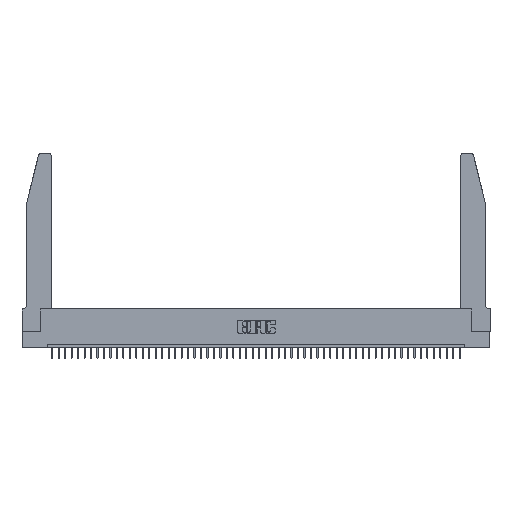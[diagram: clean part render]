
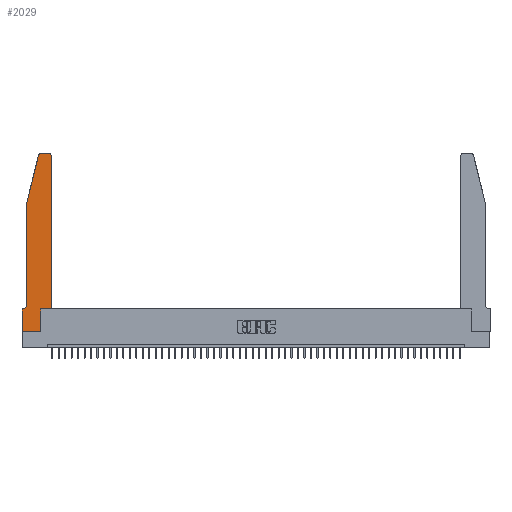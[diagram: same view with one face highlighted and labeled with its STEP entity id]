
A CAD part, top view. The second image highlights one B-rep face of the part: STEP entity #2029.
In plain terms, the highlighted planar face has unit normal (0, 0, 1).
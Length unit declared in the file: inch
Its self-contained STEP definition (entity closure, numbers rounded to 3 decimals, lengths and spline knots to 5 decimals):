
#716 = AXIS2_PLACEMENT_3D ( 'NONE', #21433, #33277, #48469 ) ;
#717 = CARTESIAN_POINT ( 'NONE',  ( 0.4505, 0.35, 0.37 ) ) ;
#1204 = AXIS2_PLACEMENT_3D ( 'NONE', #40837, #10070, #17505 ) ;
#1497 = DIRECTION ( 'NONE',  ( -0.239, -0.971, 0. ) ) ;
#2029 = ADVANCED_FACE ( 'NONE', ( #33065 ), #3967, .T. ) ;
#2465 = EDGE_CURVE ( 'NONE', #15066, #14493, #23351, .T. ) ;
#3002 = VECTOR ( 'NONE', #42410, 39.37008 ) ;
#3051 = ORIENTED_EDGE ( 'NONE', *, *, #10508, .T. ) ;
#3434 = LINE ( 'NONE', #7580, #43894 ) ;
#3967 = PLANE ( 'NONE',  #37011 ) ;
#4148 = DIRECTION ( 'NONE',  ( 1., 0., 0. ) ) ;
#4444 = DIRECTION ( 'NONE',  ( 1., 0., 0. ) ) ;
#4973 = EDGE_CURVE ( 'NONE', #5153, #47117, #19461, .T. ) ;
#5054 = CARTESIAN_POINT ( 'NONE',  ( 0.0755, 2., 0.37 ) ) ;
#5062 = EDGE_CURVE ( 'NONE', #17754, #27883, #32787, .T. ) ;
#5153 = VERTEX_POINT ( 'NONE', #25696 ) ;
#5243 = CARTESIAN_POINT ( 'NONE',  ( 0.4505, 2.72, 0.37 ) ) ;
#5812 = EDGE_CURVE ( 'NONE', #46276, #41531, #23033, .T. ) ;
#6817 = LINE ( 'NONE', #15772, #7453 ) ;
#6867 = CARTESIAN_POINT ( 'NONE',  ( 0., 0.35, 0.37 ) ) ;
#7453 = VECTOR ( 'NONE', #4148, 39.37008 ) ;
#7580 = CARTESIAN_POINT ( 'NONE',  ( 0.2865, 0.35, 0.37 ) ) ;
#7877 = EDGE_LOOP ( 'NONE', ( #15060, #33565, #18424, #22862, #23961, #18065, #3051, #20546, #26786, #35140, #23641, #13980 ) ) ;
#8109 = VECTOR ( 'NONE', #30104, 39.37008 ) ;
#9241 = CARTESIAN_POINT ( 'NONE',  ( 0.2865, 0., 0.37 ) ) ;
#9761 = VECTOR ( 'NONE', #30238, 39.37008 ) ;
#10070 = DIRECTION ( 'NONE',  ( 0., 0., 1. ) ) ;
#10508 = EDGE_CURVE ( 'NONE', #20552, #17754, #45539, .T. ) ;
#11319 = CARTESIAN_POINT ( 'NONE',  ( 0.0755, 0.35, 0.37 ) ) ;
#11421 = DIRECTION ( 'NONE',  ( 0., 1., 0. ) ) ;
#11685 = CARTESIAN_POINT ( 'NONE',  ( 0.4205, 2.75, 0.37 ) ) ;
#12059 = EDGE_CURVE ( 'NONE', #37033, #20552, #33812, .T. ) ;
#12206 = VECTOR ( 'NONE', #31632, 39.37008 ) ;
#12526 = DIRECTION ( 'NONE',  ( 0., 0., 1. ) ) ;
#13980 = ORIENTED_EDGE ( 'NONE', *, *, #49654, .T. ) ;
#14331 = AXIS2_PLACEMENT_3D ( 'NONE', #43253, #12526, #39569 ) ;
#14355 = EDGE_CURVE ( 'NONE', #41531, #37033, #35327, .T. ) ;
#14493 = VERTEX_POINT ( 'NONE', #34597 ) ;
#15060 = ORIENTED_EDGE ( 'NONE', *, *, #40405, .T. ) ;
#15066 = VERTEX_POINT ( 'NONE', #41230 ) ;
#15756 = CARTESIAN_POINT ( 'NONE',  ( 0.2865, 0.35, 0.37 ) ) ;
#15772 = CARTESIAN_POINT ( 'NONE',  ( 0.4505, 0.35, 0.37 ) ) ;
#16416 = VECTOR ( 'NONE', #36017, 39.37008 ) ;
#17505 = DIRECTION ( 'NONE',  ( 1., 0., 0. ) ) ;
#17594 = CARTESIAN_POINT ( 'NONE',  ( 0.0755, 0.42, 0.37 ) ) ;
#17754 = VERTEX_POINT ( 'NONE', #36945 ) ;
#18065 = ORIENTED_EDGE ( 'NONE', *, *, #12059, .T. ) ;
#18085 = CARTESIAN_POINT ( 'NONE',  ( 0., 0., 0.37 ) ) ;
#18424 = ORIENTED_EDGE ( 'NONE', *, *, #18780, .T. ) ;
#18780 = EDGE_CURVE ( 'NONE', #14493, #46276, #29646, .T. ) ;
#19461 = LINE ( 'NONE', #717, #12206 ) ;
#20546 = ORIENTED_EDGE ( 'NONE', *, *, #5062, .T. ) ;
#20552 = VERTEX_POINT ( 'NONE', #21061 ) ;
#21061 = CARTESIAN_POINT ( 'NONE',  ( 0., 0.35, 0.37 ) ) ;
#21070 = EDGE_CURVE ( 'NONE', #27883, #24207, #3434, .T. ) ;
#21433 = CARTESIAN_POINT ( 'NONE',  ( 0.0055, 0.42, 0.37 ) ) ;
#22862 = ORIENTED_EDGE ( 'NONE', *, *, #5812, .T. ) ;
#23033 = LINE ( 'NONE', #41065, #9761 ) ;
#23179 = CARTESIAN_POINT ( 'NONE',  ( 0.2605, 2.75, 0.37 ) ) ;
#23351 = CIRCLE ( 'NONE', #14331, 0.03 ) ;
#23486 = EDGE_CURVE ( 'NONE', #24207, #5153, #6817, .T. ) ;
#23641 = ORIENTED_EDGE ( 'NONE', *, *, #4973, .T. ) ;
#23961 = ORIENTED_EDGE ( 'NONE', *, *, #14355, .T. ) ;
#24207 = VERTEX_POINT ( 'NONE', #15756 ) ;
#25696 = CARTESIAN_POINT ( 'NONE',  ( 0.4505, 0.35, 0.37 ) ) ;
#25929 = VERTEX_POINT ( 'NONE', #11685 ) ;
#26786 = ORIENTED_EDGE ( 'NONE', *, *, #21070, .T. ) ;
#27883 = VERTEX_POINT ( 'NONE', #9241 ) ;
#27953 = CARTESIAN_POINT ( 'NONE',  ( 0.0755, 2., 0.37 ) ) ;
#29646 = LINE ( 'NONE', #5054, #48946 ) ;
#30104 = DIRECTION ( 'NONE',  ( 0., -1., 0. ) ) ;
#30238 = DIRECTION ( 'NONE',  ( 0., -1., 0. ) ) ;
#30823 = VECTOR ( 'NONE', #46492, 39.37008 ) ;
#31632 = DIRECTION ( 'NONE',  ( 0., 1., 0. ) ) ;
#32631 = CIRCLE ( 'NONE', #1204, 0.03 ) ;
#32685 = CARTESIAN_POINT ( 'NONE',  ( 0.0055, 0.35, 0.37 ) ) ;
#32787 = LINE ( 'NONE', #32802, #16416 ) ;
#32802 = CARTESIAN_POINT ( 'NONE',  ( 0., 0., 0.37 ) ) ;
#33065 = FACE_OUTER_BOUND ( 'NONE', #7877, .T. ) ;
#33277 = DIRECTION ( 'NONE',  ( 0., 0., -1. ) ) ;
#33565 = ORIENTED_EDGE ( 'NONE', *, *, #2465, .T. ) ;
#33812 = LINE ( 'NONE', #11319, #3002 ) ;
#34597 = CARTESIAN_POINT ( 'NONE',  ( 0.25487, 2.72718, 0.37 ) ) ;
#35140 = ORIENTED_EDGE ( 'NONE', *, *, #23486, .T. ) ;
#35327 = CIRCLE ( 'NONE', #716, 0.07 ) ;
#36017 = DIRECTION ( 'NONE',  ( 1., 0., 0. ) ) ;
#36945 = CARTESIAN_POINT ( 'NONE',  ( 0., 0., 0.37 ) ) ;
#37011 = AXIS2_PLACEMENT_3D ( 'NONE', #6867, #48192, #4444 ) ;
#37033 = VERTEX_POINT ( 'NONE', #32685 ) ;
#39569 = DIRECTION ( 'NONE',  ( 1., 0., 0. ) ) ;
#40405 = EDGE_CURVE ( 'NONE', #25929, #15066, #41118, .T. ) ;
#40837 = CARTESIAN_POINT ( 'NONE',  ( 0.4205, 2.72, 0.37 ) ) ;
#41065 = CARTESIAN_POINT ( 'NONE',  ( 0.0755, 2., 0.37 ) ) ;
#41118 = LINE ( 'NONE', #23179, #30823 ) ;
#41230 = CARTESIAN_POINT ( 'NONE',  ( 0.284, 2.75, 0.37 ) ) ;
#41531 = VERTEX_POINT ( 'NONE', #17594 ) ;
#42410 = DIRECTION ( 'NONE',  ( -1., 0., 0. ) ) ;
#43253 = CARTESIAN_POINT ( 'NONE',  ( 0.284, 2.72, 0.37 ) ) ;
#43894 = VECTOR ( 'NONE', #11421, 39.37008 ) ;
#45539 = LINE ( 'NONE', #18085, #8109 ) ;
#46276 = VERTEX_POINT ( 'NONE', #27953 ) ;
#46492 = DIRECTION ( 'NONE',  ( -1., 0., 0. ) ) ;
#47117 = VERTEX_POINT ( 'NONE', #5243 ) ;
#48192 = DIRECTION ( 'NONE',  ( 0., 0., 1. ) ) ;
#48469 = DIRECTION ( 'NONE',  ( -1., 0., 0. ) ) ;
#48946 = VECTOR ( 'NONE', #1497, 39.37008 ) ;
#49654 = EDGE_CURVE ( 'NONE', #47117, #25929, #32631, .T. ) ;
